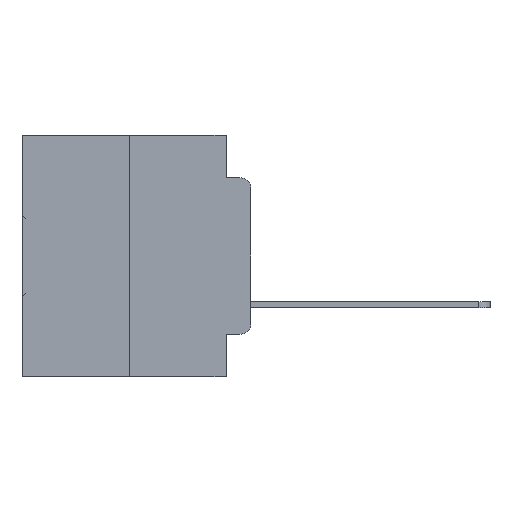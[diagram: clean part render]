
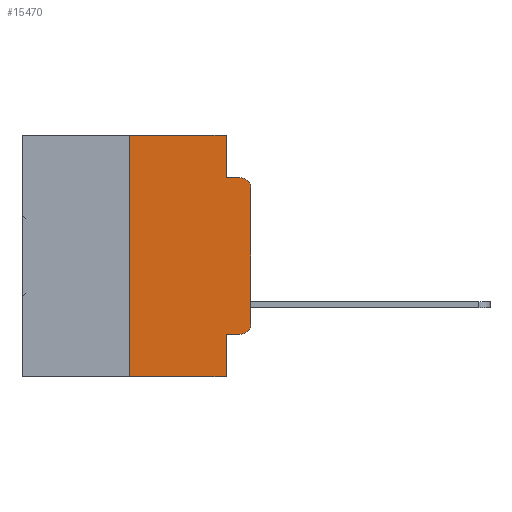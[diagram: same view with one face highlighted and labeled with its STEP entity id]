
A CAD part, left-side view. The second image highlights one B-rep face of the part: STEP entity #15470.
In plain terms, the highlighted planar face has unit normal (-1, 0, 0).
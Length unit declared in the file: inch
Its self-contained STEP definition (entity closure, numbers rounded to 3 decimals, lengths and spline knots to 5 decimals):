
#1583 = DIRECTION ( 'NONE',  ( 0., 0., 1. ) ) ;
#1638 = ORIENTED_EDGE ( 'NONE', *, *, #19717, .T. ) ;
#1875 = VERTEX_POINT ( 'NONE', #3077 ) ;
#2071 = AXIS2_PLACEMENT_3D ( 'NONE', #13474, #23893, #7960 ) ;
#2458 = AXIS2_PLACEMENT_3D ( 'NONE', #16681, #34029, #19268 ) ;
#2799 = CARTESIAN_POINT ( 'NONE',  ( 0., 0.051, -0.5 ) ) ;
#2864 = EDGE_CURVE ( 'NONE', #26353, #19548, #10719, .T. ) ;
#3034 = EDGE_CURVE ( 'NONE', #28696, #21969, #32138, .T. ) ;
#3077 = CARTESIAN_POINT ( 'NONE',  ( 0., 0., -0.1085 ) ) ;
#3552 = CARTESIAN_POINT ( 'NONE',  ( 0., 0.473, 0. ) ) ;
#3629 = DIRECTION ( 'NONE',  ( 0., 0., 1. ) ) ;
#4752 = CARTESIAN_POINT ( 'NONE',  ( 0., 0.051, 0. ) ) ;
#4821 = DIRECTION ( 'NONE',  ( 0., -1., 0. ) ) ;
#4881 = LINE ( 'NONE', #11078, #31813 ) ;
#5018 = PLANE ( 'NONE',  #2071 ) ;
#6046 = CARTESIAN_POINT ( 'NONE',  ( 0., 0.051, -0.4115 ) ) ;
#6126 = ORIENTED_EDGE ( 'NONE', *, *, #18010, .T. ) ;
#6834 = CARTESIAN_POINT ( 'NONE',  ( 0., 0.051, 0. ) ) ;
#7004 = EDGE_CURVE ( 'NONE', #9530, #26353, #18837, .T. ) ;
#7191 = LINE ( 'NONE', #32074, #14616 ) ;
#7226 = VERTEX_POINT ( 'NONE', #31126 ) ;
#7960 = DIRECTION ( 'NONE',  ( 0., 0., -1. ) ) ;
#8939 = EDGE_CURVE ( 'NONE', #19548, #19884, #7191, .T. ) ;
#9530 = VERTEX_POINT ( 'NONE', #22334 ) ;
#9815 = VECTOR ( 'NONE', #4821, 39.37008 ) ;
#9909 = EDGE_CURVE ( 'NONE', #9530, #21969, #4881, .T. ) ;
#10719 = LINE ( 'NONE', #3552, #9815 ) ;
#11078 = CARTESIAN_POINT ( 'NONE',  ( 0., 0.473, -0.5 ) ) ;
#11369 = ORIENTED_EDGE ( 'NONE', *, *, #3034, .F. ) ;
#11397 = DIRECTION ( 'NONE',  ( -1., 0., 0. ) ) ;
#11513 = LINE ( 'NONE', #28360, #24575 ) ;
#12665 = VECTOR ( 'NONE', #3629, 39.37008 ) ;
#13474 = CARTESIAN_POINT ( 'NONE',  ( 0., 0.473, 0. ) ) ;
#13603 = ORIENTED_EDGE ( 'NONE', *, *, #9909, .T. ) ;
#14616 = VECTOR ( 'NONE', #17239, 39.37008 ) ;
#14757 = ORIENTED_EDGE ( 'NONE', *, *, #16244, .F. ) ;
#15404 = CARTESIAN_POINT ( 'NONE',  ( 0., 0.02, -0.4115 ) ) ;
#15470 = ADVANCED_FACE ( 'NONE', ( #22711 ), #5018, .F. ) ;
#16244 = EDGE_CURVE ( 'NONE', #19884, #26578, #17151, .T. ) ;
#16681 = CARTESIAN_POINT ( 'NONE',  ( 0., 0.02, -0.3915 ) ) ;
#17151 = LINE ( 'NONE', #24300, #29655 ) ;
#17239 = DIRECTION ( 'NONE',  ( 0., 0., -1. ) ) ;
#18010 = EDGE_CURVE ( 'NONE', #1875, #26578, #22650, .T. ) ;
#18762 = ORIENTED_EDGE ( 'NONE', *, *, #2864, .F. ) ;
#18837 = LINE ( 'NONE', #22693, #12665 ) ;
#19075 = DIRECTION ( 'NONE',  ( 0., -1., 0. ) ) ;
#19268 = DIRECTION ( 'NONE',  ( 0., 0., -1. ) ) ;
#19548 = VERTEX_POINT ( 'NONE', #6834 ) ;
#19717 = EDGE_CURVE ( 'NONE', #7226, #1875, #11513, .T. ) ;
#19884 = VERTEX_POINT ( 'NONE', #28976 ) ;
#21303 = ORIENTED_EDGE ( 'NONE', *, *, #8939, .F. ) ;
#21559 = ORIENTED_EDGE ( 'NONE', *, *, #30292, .T. ) ;
#21969 = VERTEX_POINT ( 'NONE', #2799 ) ;
#22334 = CARTESIAN_POINT ( 'NONE',  ( 0., 0.25, -0.5 ) ) ;
#22650 = CIRCLE ( 'NONE', #33301, 0.02 ) ;
#22693 = CARTESIAN_POINT ( 'NONE',  ( 0., 0.25, 0. ) ) ;
#22711 = FACE_OUTER_BOUND ( 'NONE', #31419, .T. ) ;
#23304 = VERTEX_POINT ( 'NONE', #15404 ) ;
#23893 = DIRECTION ( 'NONE',  ( 1., 0., 0. ) ) ;
#24234 = VECTOR ( 'NONE', #26400, 39.37008 ) ;
#24300 = CARTESIAN_POINT ( 'NONE',  ( 0., 0.051, -0.0885 ) ) ;
#24575 = VECTOR ( 'NONE', #1583, 39.37008 ) ;
#25546 = CARTESIAN_POINT ( 'NONE',  ( 0., 0.25, 0. ) ) ;
#26353 = VERTEX_POINT ( 'NONE', #25546 ) ;
#26400 = DIRECTION ( 'NONE',  ( 0., 0., -1. ) ) ;
#26578 = VERTEX_POINT ( 'NONE', #30067 ) ;
#26644 = ORIENTED_EDGE ( 'NONE', *, *, #7004, .F. ) ;
#26833 = CARTESIAN_POINT ( 'NONE',  ( 0., 0.02, -0.1085 ) ) ;
#28360 = CARTESIAN_POINT ( 'NONE',  ( 0., 0., 0. ) ) ;
#28696 = VERTEX_POINT ( 'NONE', #6046 ) ;
#28726 = VECTOR ( 'NONE', #32574, 39.37008 ) ;
#28976 = CARTESIAN_POINT ( 'NONE',  ( 0., 0.051, -0.0885 ) ) ;
#29231 = CIRCLE ( 'NONE', #2458, 0.02 ) ;
#29265 = DIRECTION ( 'NONE',  ( 0., 0., -1. ) ) ;
#29655 = VECTOR ( 'NONE', #31563, 39.37008 ) ;
#30067 = CARTESIAN_POINT ( 'NONE',  ( 0., 0.02, -0.0885 ) ) ;
#30180 = CARTESIAN_POINT ( 'NONE',  ( 0., 0.051, -0.4115 ) ) ;
#30242 = LINE ( 'NONE', #30180, #28726 ) ;
#30292 = EDGE_CURVE ( 'NONE', #23304, #7226, #29231, .T. ) ;
#31126 = CARTESIAN_POINT ( 'NONE',  ( 0., 0., -0.3915 ) ) ;
#31419 = EDGE_LOOP ( 'NONE', ( #1638, #6126, #14757, #21303, #18762, #26644, #13603, #11369, #31552, #21559 ) ) ;
#31552 = ORIENTED_EDGE ( 'NONE', *, *, #33523, .T. ) ;
#31563 = DIRECTION ( 'NONE',  ( 0., -1., 0. ) ) ;
#31813 = VECTOR ( 'NONE', #19075, 39.37008 ) ;
#32074 = CARTESIAN_POINT ( 'NONE',  ( 0., 0.051, 0. ) ) ;
#32138 = LINE ( 'NONE', #4752, #24234 ) ;
#32574 = DIRECTION ( 'NONE',  ( 0., -1., 0. ) ) ;
#33301 = AXIS2_PLACEMENT_3D ( 'NONE', #26833, #11397, #29265 ) ;
#33523 = EDGE_CURVE ( 'NONE', #28696, #23304, #30242, .T. ) ;
#34029 = DIRECTION ( 'NONE',  ( -1., 0., 0. ) ) ;
